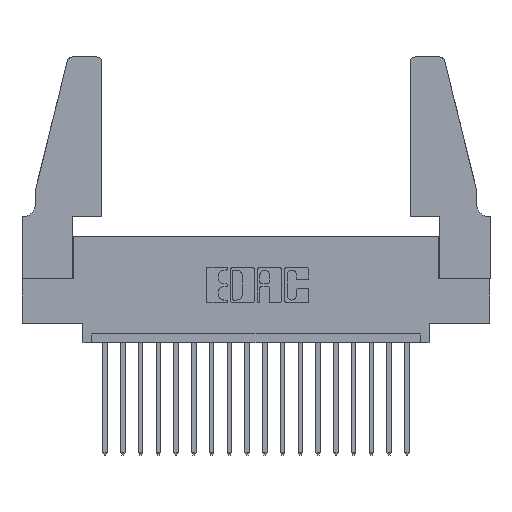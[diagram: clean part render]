
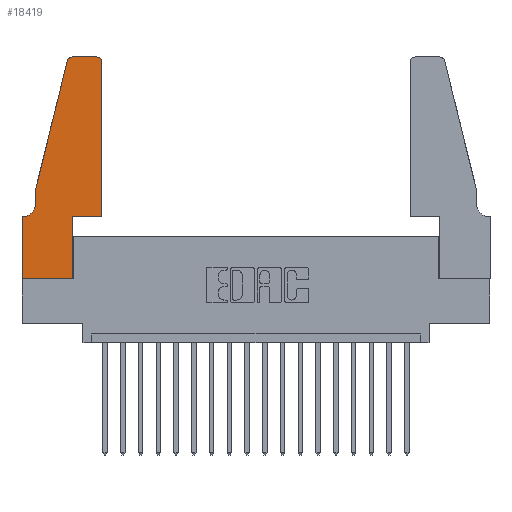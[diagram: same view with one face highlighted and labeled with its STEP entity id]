
A CAD part, top view. The second image highlights one B-rep face of the part: STEP entity #18419.
In plain terms, the highlighted planar face has unit normal (0, 0, 1).
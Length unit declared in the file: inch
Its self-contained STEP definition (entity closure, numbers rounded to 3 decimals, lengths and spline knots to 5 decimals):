
#122 = CARTESIAN_POINT ( 'NONE',  ( 0.4205, 1.25, 0.37 ) ) ;
#137 = CIRCLE ( 'NONE', #11124, 0.07 ) ;
#186 = EDGE_CURVE ( 'NONE', #15006, #15015, #1476, .T. ) ;
#199 = LINE ( 'NONE', #13548, #2992 ) ;
#517 = LINE ( 'NONE', #7312, #17784 ) ;
#602 = ORIENTED_EDGE ( 'NONE', *, *, #9637, .T. ) ;
#624 = VECTOR ( 'NONE', #16815, 39.37008 ) ;
#723 = EDGE_CURVE ( 'NONE', #17263, #10650, #18732, .T. ) ;
#747 = DIRECTION ( 'NONE',  ( -1., 0., 0. ) ) ;
#1476 = LINE ( 'NONE', #3774, #9529 ) ;
#1493 = EDGE_LOOP ( 'NONE', ( #3976, #602, #16670, #15731, #17043, #9163, #13401, #6678, #10632, #18542, #14942, #9428 ) ) ;
#2049 = CARTESIAN_POINT ( 'NONE',  ( 0.2865, 0.35, 0.37 ) ) ;
#2051 = VECTOR ( 'NONE', #13802, 39.37008 ) ;
#2548 = DIRECTION ( 'NONE',  ( -1., 0., 0. ) ) ;
#2992 = VECTOR ( 'NONE', #6221, 39.37008 ) ;
#3409 = CARTESIAN_POINT ( 'NONE',  ( 0.2865, 0., 0.37 ) ) ;
#3774 = CARTESIAN_POINT ( 'NONE',  ( 0.0755, 0.35, 0.37 ) ) ;
#3976 = ORIENTED_EDGE ( 'NONE', *, *, #723, .T. ) ;
#4020 = DIRECTION ( 'NONE',  ( 0., 0., 1. ) ) ;
#4183 = CARTESIAN_POINT ( 'NONE',  ( 0.4505, 0.35, 0.37 ) ) ;
#4254 = LINE ( 'NONE', #9968, #6066 ) ;
#5068 = CARTESIAN_POINT ( 'NONE',  ( 0.284, 1.25, 0.37 ) ) ;
#5214 = DIRECTION ( 'NONE',  ( -0.239, -0.971, 0. ) ) ;
#5278 = CARTESIAN_POINT ( 'NONE',  ( 0.0755, 0.5, 0.37 ) ) ;
#5605 = AXIS2_PLACEMENT_3D ( 'NONE', #12475, #14005, #11252 ) ;
#5937 = VERTEX_POINT ( 'NONE', #13493 ) ;
#5991 = CARTESIAN_POINT ( 'NONE',  ( 0., 0., 0.37 ) ) ;
#6066 = VECTOR ( 'NONE', #6925, 39.37008 ) ;
#6131 = LINE ( 'NONE', #2049, #624 ) ;
#6204 = CARTESIAN_POINT ( 'NONE',  ( 0., 0., 0.37 ) ) ;
#6221 = DIRECTION ( 'NONE',  ( 1., 0., 0. ) ) ;
#6678 = ORIENTED_EDGE ( 'NONE', *, *, #13719, .T. ) ;
#6811 = CARTESIAN_POINT ( 'NONE',  ( 0.0755, 0.5, 0.37 ) ) ;
#6925 = DIRECTION ( 'NONE',  ( 0., -1., 0. ) ) ;
#6995 = LINE ( 'NONE', #4183, #9316 ) ;
#7312 = CARTESIAN_POINT ( 'NONE',  ( 0.4505, 0.35, 0.37 ) ) ;
#7532 = DIRECTION ( 'NONE',  ( 1., 0., 0. ) ) ;
#7621 = EDGE_CURVE ( 'NONE', #18507, #18679, #4254, .T. ) ;
#7625 = DIRECTION ( 'NONE',  ( 0., 1., 0. ) ) ;
#8268 = CARTESIAN_POINT ( 'NONE',  ( 0.0055, 0.35, 0.37 ) ) ;
#8291 = EDGE_CURVE ( 'NONE', #13191, #10959, #6995, .T. ) ;
#8377 = FACE_OUTER_BOUND ( 'NONE', #1493, .T. ) ;
#8716 = CARTESIAN_POINT ( 'NONE',  ( 0.4205, 1.22, 0.37 ) ) ;
#9047 = CARTESIAN_POINT ( 'NONE',  ( 0.2605, 1.25, 0.37 ) ) ;
#9108 = VERTEX_POINT ( 'NONE', #5991 ) ;
#9163 = ORIENTED_EDGE ( 'NONE', *, *, #186, .T. ) ;
#9316 = VECTOR ( 'NONE', #7532, 39.37008 ) ;
#9428 = ORIENTED_EDGE ( 'NONE', *, *, #15114, .T. ) ;
#9529 = VECTOR ( 'NONE', #747, 39.37008 ) ;
#9637 = EDGE_CURVE ( 'NONE', #10650, #9838, #17046, .T. ) ;
#9779 = CARTESIAN_POINT ( 'NONE',  ( 0.4505, 0.35, 0.37 ) ) ;
#9838 = VERTEX_POINT ( 'NONE', #9859 ) ;
#9859 = CARTESIAN_POINT ( 'NONE',  ( 0.25487, 1.22718, 0.37 ) ) ;
#9968 = CARTESIAN_POINT ( 'NONE',  ( 0.0755, 0.5, 0.37 ) ) ;
#10039 = DIRECTION ( 'NONE',  ( 1., 0., 0. ) ) ;
#10073 = VERTEX_POINT ( 'NONE', #3409 ) ;
#10632 = ORIENTED_EDGE ( 'NONE', *, *, #11977, .T. ) ;
#10650 = VERTEX_POINT ( 'NONE', #5068 ) ;
#10791 = CIRCLE ( 'NONE', #13551, 0.03 ) ;
#10959 = VERTEX_POINT ( 'NONE', #9779 ) ;
#11029 = VECTOR ( 'NONE', #5214, 39.37008 ) ;
#11124 = AXIS2_PLACEMENT_3D ( 'NONE', #12771, #17199, #2548 ) ;
#11252 = DIRECTION ( 'NONE',  ( 1., 0., 0. ) ) ;
#11546 = DIRECTION ( 'NONE',  ( 1., 0., 0. ) ) ;
#11977 = EDGE_CURVE ( 'NONE', #10073, #13191, #6131, .T. ) ;
#12010 = CARTESIAN_POINT ( 'NONE',  ( 0.0755, 0.42, 0.37 ) ) ;
#12475 = CARTESIAN_POINT ( 'NONE',  ( 0., 0.35, 0.37 ) ) ;
#12620 = EDGE_CURVE ( 'NONE', #10959, #5937, #517, .T. ) ;
#12657 = PLANE ( 'NONE',  #5605 ) ;
#12771 = CARTESIAN_POINT ( 'NONE',  ( 0.0055, 0.42, 0.37 ) ) ;
#13191 = VERTEX_POINT ( 'NONE', #16741 ) ;
#13401 = ORIENTED_EDGE ( 'NONE', *, *, #14395, .T. ) ;
#13493 = CARTESIAN_POINT ( 'NONE',  ( 0.4505, 1.22, 0.37 ) ) ;
#13548 = CARTESIAN_POINT ( 'NONE',  ( 0., 0., 0.37 ) ) ;
#13551 = AXIS2_PLACEMENT_3D ( 'NONE', #8716, #4020, #11546 ) ;
#13578 = DIRECTION ( 'NONE',  ( -1., 0., 0. ) ) ;
#13719 = EDGE_CURVE ( 'NONE', #9108, #10073, #199, .T. ) ;
#13802 = DIRECTION ( 'NONE',  ( 0., -1., 0. ) ) ;
#13863 = VECTOR ( 'NONE', #13578, 39.37008 ) ;
#14005 = DIRECTION ( 'NONE',  ( 0., 0., 1. ) ) ;
#14395 = EDGE_CURVE ( 'NONE', #15015, #9108, #17704, .T. ) ;
#14818 = EDGE_CURVE ( 'NONE', #9838, #18507, #14913, .T. ) ;
#14913 = LINE ( 'NONE', #5278, #11029 ) ;
#14942 = ORIENTED_EDGE ( 'NONE', *, *, #12620, .T. ) ;
#15006 = VERTEX_POINT ( 'NONE', #8268 ) ;
#15015 = VERTEX_POINT ( 'NONE', #16981 ) ;
#15114 = EDGE_CURVE ( 'NONE', #5937, #17263, #10791, .T. ) ;
#15525 = EDGE_CURVE ( 'NONE', #18679, #15006, #137, .T. ) ;
#15731 = ORIENTED_EDGE ( 'NONE', *, *, #7621, .T. ) ;
#16670 = ORIENTED_EDGE ( 'NONE', *, *, #14818, .T. ) ;
#16741 = CARTESIAN_POINT ( 'NONE',  ( 0.2865, 0.35, 0.37 ) ) ;
#16815 = DIRECTION ( 'NONE',  ( 0., 1., 0. ) ) ;
#16981 = CARTESIAN_POINT ( 'NONE',  ( 0., 0.35, 0.37 ) ) ;
#17043 = ORIENTED_EDGE ( 'NONE', *, *, #15525, .T. ) ;
#17046 = CIRCLE ( 'NONE', #18699, 0.03 ) ;
#17199 = DIRECTION ( 'NONE',  ( 0., 0., -1. ) ) ;
#17263 = VERTEX_POINT ( 'NONE', #122 ) ;
#17704 = LINE ( 'NONE', #6204, #2051 ) ;
#17784 = VECTOR ( 'NONE', #7625, 39.37008 ) ;
#18419 = ADVANCED_FACE ( 'NONE', ( #8377 ), #12657, .T. ) ;
#18507 = VERTEX_POINT ( 'NONE', #6811 ) ;
#18542 = ORIENTED_EDGE ( 'NONE', *, *, #8291, .T. ) ;
#18679 = VERTEX_POINT ( 'NONE', #12010 ) ;
#18699 = AXIS2_PLACEMENT_3D ( 'NONE', #18762, #18954, #10039 ) ;
#18732 = LINE ( 'NONE', #9047, #13863 ) ;
#18762 = CARTESIAN_POINT ( 'NONE',  ( 0.284, 1.22, 0.37 ) ) ;
#18954 = DIRECTION ( 'NONE',  ( 0., 0., 1. ) ) ;
